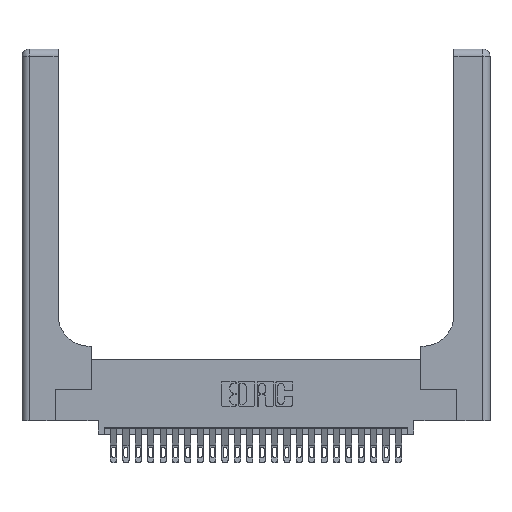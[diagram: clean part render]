
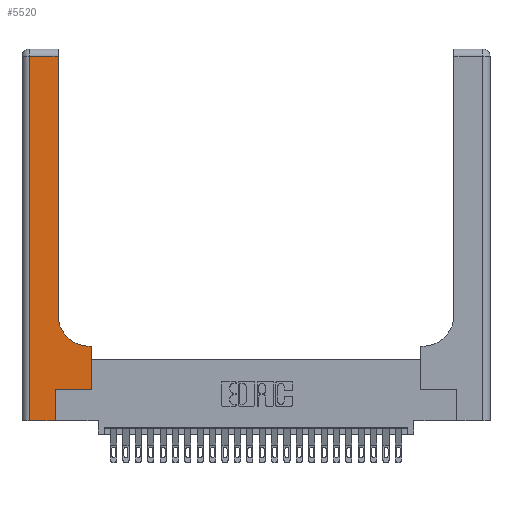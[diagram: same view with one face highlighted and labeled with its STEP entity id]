
A CAD part, top view. The second image highlights one B-rep face of the part: STEP entity #5520.
In plain terms, the highlighted planar face has unit normal (0, 0, 1).
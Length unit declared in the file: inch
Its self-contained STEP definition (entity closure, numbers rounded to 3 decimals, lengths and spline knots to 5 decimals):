
#290 = VECTOR ( 'NONE', #8264, 39.37008 ) ;
#881 = CARTESIAN_POINT ( 'NONE',  ( 0.269, 0., 0.37 ) ) ;
#1075 = ORIENTED_EDGE ( 'NONE', *, *, #4909, .T. ) ;
#1241 = EDGE_CURVE ( 'NONE', #18670, #6792, #13139, .T. ) ;
#1875 = DIRECTION ( 'NONE',  ( -1., 0., 0. ) ) ;
#1894 = CARTESIAN_POINT ( 'NONE',  ( 0.269, 0.25, 0.37 ) ) ;
#1947 = VECTOR ( 'NONE', #15189, 39.37008 ) ;
#2338 = EDGE_CURVE ( 'NONE', #17870, #23070, #11485, .T. ) ;
#2696 = EDGE_CURVE ( 'NONE', #6792, #17870, #2921, .T. ) ;
#2858 = EDGE_LOOP ( 'NONE', ( #4732, #1075, #12591, #21353, #24909, #21734, #18577, #5515, #12175 ) ) ;
#2921 = LINE ( 'NONE', #881, #24363 ) ;
#3096 = CARTESIAN_POINT ( 'NONE',  ( 0.2915, 3., 0.37 ) ) ;
#3687 = CARTESIAN_POINT ( 'NONE',  ( 0., 3., 0.37 ) ) ;
#3917 = VERTEX_POINT ( 'NONE', #17665 ) ;
#4283 = CARTESIAN_POINT ( 'NONE',  ( 0.2915, 0.85, 0.37 ) ) ;
#4508 = CARTESIAN_POINT ( 'NONE',  ( 0.06, 3., 0.37 ) ) ;
#4732 = ORIENTED_EDGE ( 'NONE', *, *, #23719, .T. ) ;
#4803 = AXIS2_PLACEMENT_3D ( 'NONE', #18240, #5744, #20311 ) ;
#4909 = EDGE_CURVE ( 'NONE', #3917, #6570, #25490, .T. ) ;
#5351 = CARTESIAN_POINT ( 'NONE',  ( 0.5585, 0.25, 0.37 ) ) ;
#5515 = ORIENTED_EDGE ( 'NONE', *, *, #13762, .T. ) ;
#5520 = ADVANCED_FACE ( 'NONE', ( #12963 ), #10022, .F. ) ;
#5668 = EDGE_CURVE ( 'NONE', #6570, #18670, #20074, .T. ) ;
#5744 = DIRECTION ( 'NONE',  ( 0., 0., -1. ) ) ;
#5925 = LINE ( 'NONE', #3096, #21855 ) ;
#6145 = DIRECTION ( 'NONE',  ( 0., 1., 0. ) ) ;
#6570 = VERTEX_POINT ( 'NONE', #13617 ) ;
#6591 = CARTESIAN_POINT ( 'NONE',  ( 0.269, 0.25, 0.37 ) ) ;
#6792 = VERTEX_POINT ( 'NONE', #26819 ) ;
#6893 = VERTEX_POINT ( 'NONE', #4283 ) ;
#7119 = DIRECTION ( 'NONE',  ( -1., 0., 0. ) ) ;
#8234 = VERTEX_POINT ( 'NONE', #21698 ) ;
#8264 = DIRECTION ( 'NONE',  ( 1., 0., 0. ) ) ;
#8370 = LINE ( 'NONE', #12376, #18158 ) ;
#9017 = VECTOR ( 'NONE', #7119, 39.37008 ) ;
#9129 = EDGE_CURVE ( 'NONE', #12882, #6893, #9150, .T. ) ;
#9150 = CIRCLE ( 'NONE', #4803, 0.25 ) ;
#10022 = PLANE ( 'NONE',  #26730 ) ;
#11253 = CARTESIAN_POINT ( 'NONE',  ( 0.06, 0., 0.37 ) ) ;
#11485 = LINE ( 'NONE', #1894, #290 ) ;
#11682 = CARTESIAN_POINT ( 'NONE',  ( 0.5415, 0.6, 0.37 ) ) ;
#12123 = DIRECTION ( 'NONE',  ( 0., 0., -1. ) ) ;
#12175 = ORIENTED_EDGE ( 'NONE', *, *, #9129, .T. ) ;
#12376 = CARTESIAN_POINT ( 'NONE',  ( 0.5585, 0.25, 0.37 ) ) ;
#12591 = ORIENTED_EDGE ( 'NONE', *, *, #5668, .T. ) ;
#12832 = DIRECTION ( 'NONE',  ( 0., -1., 0. ) ) ;
#12882 = VERTEX_POINT ( 'NONE', #11682 ) ;
#12963 = FACE_OUTER_BOUND ( 'NONE', #2858, .T. ) ;
#13082 = CARTESIAN_POINT ( 'NONE',  ( 0., 0., 0.37 ) ) ;
#13139 = LINE ( 'NONE', #13082, #1947 ) ;
#13617 = CARTESIAN_POINT ( 'NONE',  ( 0.06, 2.94, 0.37 ) ) ;
#13646 = DIRECTION ( 'NONE',  ( 0., 1., 0. ) ) ;
#13762 = EDGE_CURVE ( 'NONE', #8234, #12882, #23665, .T. ) ;
#13940 = VECTOR ( 'NONE', #12832, 39.37008 ) ;
#14479 = CARTESIAN_POINT ( 'NONE',  ( 0.2915, 0.6, 0.37 ) ) ;
#15189 = DIRECTION ( 'NONE',  ( 1., 0., 0. ) ) ;
#15424 = CARTESIAN_POINT ( 'NONE',  ( 0., 2.94, 0.37 ) ) ;
#17665 = CARTESIAN_POINT ( 'NONE',  ( 0.2915, 2.94, 0.37 ) ) ;
#17870 = VERTEX_POINT ( 'NONE', #6591 ) ;
#18158 = VECTOR ( 'NONE', #6145, 39.37008 ) ;
#18240 = CARTESIAN_POINT ( 'NONE',  ( 0.5415, 0.85, 0.37 ) ) ;
#18577 = ORIENTED_EDGE ( 'NONE', *, *, #26811, .T. ) ;
#18670 = VERTEX_POINT ( 'NONE', #11253 ) ;
#20074 = LINE ( 'NONE', #4508, #13940 ) ;
#20311 = DIRECTION ( 'NONE',  ( 1., 0., 0. ) ) ;
#21353 = ORIENTED_EDGE ( 'NONE', *, *, #1241, .T. ) ;
#21698 = CARTESIAN_POINT ( 'NONE',  ( 0.5585, 0.6, 0.37 ) ) ;
#21734 = ORIENTED_EDGE ( 'NONE', *, *, #2338, .T. ) ;
#21780 = DIRECTION ( 'NONE',  ( 0., 1., 0. ) ) ;
#21855 = VECTOR ( 'NONE', #13646, 39.37008 ) ;
#23070 = VERTEX_POINT ( 'NONE', #5351 ) ;
#23665 = LINE ( 'NONE', #14479, #24307 ) ;
#23719 = EDGE_CURVE ( 'NONE', #6893, #3917, #5925, .T. ) ;
#24307 = VECTOR ( 'NONE', #1875, 39.37008 ) ;
#24363 = VECTOR ( 'NONE', #21780, 39.37008 ) ;
#24909 = ORIENTED_EDGE ( 'NONE', *, *, #2696, .T. ) ;
#25490 = LINE ( 'NONE', #15424, #9017 ) ;
#26507 = DIRECTION ( 'NONE',  ( -1., 0., 0. ) ) ;
#26730 = AXIS2_PLACEMENT_3D ( 'NONE', #3687, #12123, #26507 ) ;
#26811 = EDGE_CURVE ( 'NONE', #23070, #8234, #8370, .T. ) ;
#26819 = CARTESIAN_POINT ( 'NONE',  ( 0.269, 0., 0.37 ) ) ;
